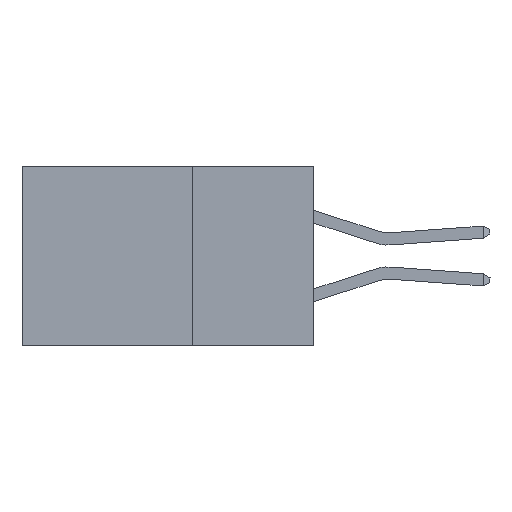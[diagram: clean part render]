
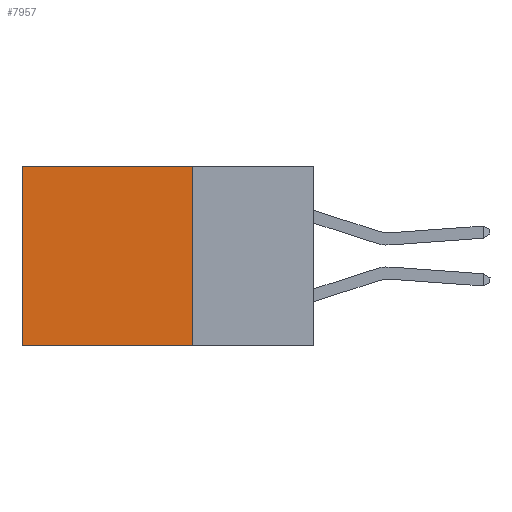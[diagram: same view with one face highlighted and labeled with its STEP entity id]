
A CAD part, left-side view. The second image highlights one B-rep face of the part: STEP entity #7957.
In plain terms, the highlighted planar face has unit normal (-1, 0, 0).
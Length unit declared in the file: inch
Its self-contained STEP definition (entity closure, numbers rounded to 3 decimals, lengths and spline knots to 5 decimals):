
#337 = DIRECTION ( 'NONE',  ( 0., 0., -1. ) ) ;
#426 = DIRECTION ( 'NONE',  ( 0., 1., 0. ) ) ;
#430 = CARTESIAN_POINT ( 'NONE',  ( 0.2875, 0.25, 0. ) ) ;
#547 = LINE ( 'NONE', #9499, #8945 ) ;
#1051 = ORIENTED_EDGE ( 'NONE', *, *, #5672, .F. ) ;
#1322 = CARTESIAN_POINT ( 'NONE',  ( 0.2875, 0.25, 0. ) ) ;
#2098 = VECTOR ( 'NONE', #426, 39.37008 ) ;
#2302 = EDGE_CURVE ( 'NONE', #11443, #9712, #11020, .T. ) ;
#2464 = EDGE_LOOP ( 'NONE', ( #6014, #1051, #7228, #3139 ) ) ;
#2647 = CARTESIAN_POINT ( 'NONE',  ( 0.2875, 0.6, 0. ) ) ;
#2879 = DIRECTION ( 'NONE',  ( 0., 0., -1. ) ) ;
#3139 = ORIENTED_EDGE ( 'NONE', *, *, #6308, .T. ) ;
#4073 = VERTEX_POINT ( 'NONE', #7733 ) ;
#4111 = EDGE_CURVE ( 'NONE', #9137, #4073, #4808, .T. ) ;
#4637 = LINE ( 'NONE', #7607, #2098 ) ;
#4808 = LINE ( 'NONE', #8683, #9259 ) ;
#5370 = AXIS2_PLACEMENT_3D ( 'NONE', #430, #5726, #337 ) ;
#5622 = FACE_OUTER_BOUND ( 'NONE', #2464, .T. ) ;
#5672 = EDGE_CURVE ( 'NONE', #9712, #4073, #4637, .T. ) ;
#5726 = DIRECTION ( 'NONE',  ( 1., 0., 0. ) ) ;
#5742 = CARTESIAN_POINT ( 'NONE',  ( 0.2875, 0.25, -0.37 ) ) ;
#5963 = DIRECTION ( 'NONE',  ( 0., 1., 0. ) ) ;
#6014 = ORIENTED_EDGE ( 'NONE', *, *, #4111, .T. ) ;
#6026 = DIRECTION ( 'NONE',  ( 0., 0., -1. ) ) ;
#6308 = EDGE_CURVE ( 'NONE', #11443, #9137, #547, .T. ) ;
#7228 = ORIENTED_EDGE ( 'NONE', *, *, #2302, .F. ) ;
#7238 = VECTOR ( 'NONE', #2879, 39.37008 ) ;
#7607 = CARTESIAN_POINT ( 'NONE',  ( 0.2875, 0.25, -0.37 ) ) ;
#7733 = CARTESIAN_POINT ( 'NONE',  ( 0.2875, 0.6, -0.37 ) ) ;
#7957 = ADVANCED_FACE ( 'NONE', ( #5622 ), #10164, .F. ) ;
#8683 = CARTESIAN_POINT ( 'NONE',  ( 0.2875, 0.6, 0. ) ) ;
#8945 = VECTOR ( 'NONE', #5963, 39.37008 ) ;
#9100 = CARTESIAN_POINT ( 'NONE',  ( 0.2875, 0.25, 0. ) ) ;
#9137 = VERTEX_POINT ( 'NONE', #2647 ) ;
#9259 = VECTOR ( 'NONE', #6026, 39.37008 ) ;
#9499 = CARTESIAN_POINT ( 'NONE',  ( 0.2875, 0.25, 0. ) ) ;
#9712 = VERTEX_POINT ( 'NONE', #5742 ) ;
#10164 = PLANE ( 'NONE',  #5370 ) ;
#11020 = LINE ( 'NONE', #9100, #7238 ) ;
#11443 = VERTEX_POINT ( 'NONE', #1322 ) ;
